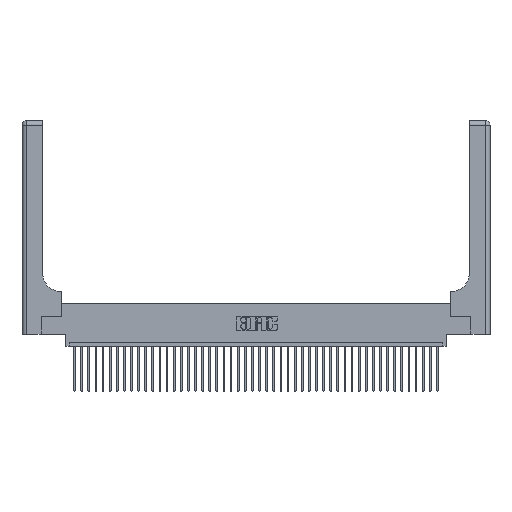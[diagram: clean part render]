
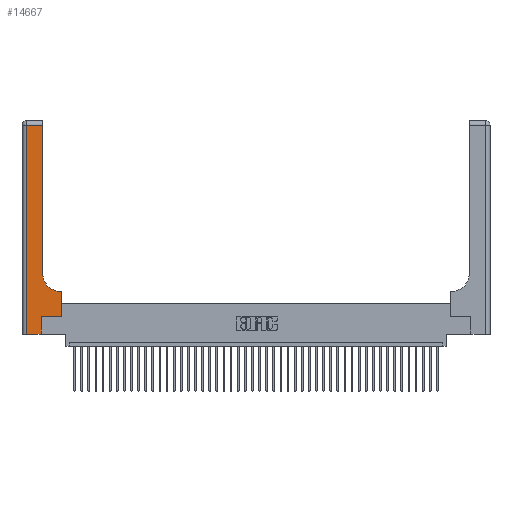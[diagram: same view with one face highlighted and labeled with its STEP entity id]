
A CAD part, top view. The second image highlights one B-rep face of the part: STEP entity #14667.
In plain terms, the highlighted planar face has unit normal (0, 0, 1).
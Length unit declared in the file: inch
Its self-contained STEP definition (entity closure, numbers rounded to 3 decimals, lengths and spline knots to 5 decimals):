
#72 = EDGE_CURVE ( 'NONE', #27932, #22813, #7140, .T. ) ;
#985 = CARTESIAN_POINT ( 'NONE',  ( 0.5585, 0.6, 0.37 ) ) ;
#1451 = VECTOR ( 'NONE', #40873, 39.37008 ) ;
#1504 = EDGE_CURVE ( 'NONE', #22813, #14280, #8619, .T. ) ;
#2608 = CARTESIAN_POINT ( 'NONE',  ( 0.5415, 0.6, 0.37 ) ) ;
#3847 = LINE ( 'NONE', #9476, #41307 ) ;
#5202 = EDGE_CURVE ( 'NONE', #39440, #27932, #33049, .T. ) ;
#6873 = CARTESIAN_POINT ( 'NONE',  ( 0.2915, 3., 0.37 ) ) ;
#7140 = CIRCLE ( 'NONE', #28200, 0.25 ) ;
#8091 = CARTESIAN_POINT ( 'NONE',  ( 0., 2.94, 0.37 ) ) ;
#8465 = DIRECTION ( 'NONE',  ( 1., 0., 0. ) ) ;
#8619 = LINE ( 'NONE', #6873, #30538 ) ;
#9246 = DIRECTION ( 'NONE',  ( 0., 1., 0. ) ) ;
#9343 = CARTESIAN_POINT ( 'NONE',  ( 0.5585, 0.25, 0.37 ) ) ;
#9476 = CARTESIAN_POINT ( 'NONE',  ( 0.5585, 0.25, 0.37 ) ) ;
#10538 = EDGE_LOOP ( 'NONE', ( #39473, #32038, #26495, #14213, #32783, #10696, #21372, #36555, #38969 ) ) ;
#10696 = ORIENTED_EDGE ( 'NONE', *, *, #23498, .T. ) ;
#11428 = CARTESIAN_POINT ( 'NONE',  ( 0.2915, 0.85, 0.37 ) ) ;
#12403 = AXIS2_PLACEMENT_3D ( 'NONE', #36168, #19683, #12734 ) ;
#12734 = DIRECTION ( 'NONE',  ( -1., 0., 0. ) ) ;
#14213 = ORIENTED_EDGE ( 'NONE', *, *, #15661, .T. ) ;
#14280 = VERTEX_POINT ( 'NONE', #30694 ) ;
#14667 = ADVANCED_FACE ( 'NONE', ( #39148 ), #19255, .F. ) ;
#14731 = CARTESIAN_POINT ( 'NONE',  ( 0.06, 3., 0.37 ) ) ;
#14767 = VERTEX_POINT ( 'NONE', #30352 ) ;
#15527 = CARTESIAN_POINT ( 'NONE',  ( 0.269, 0., 0.37 ) ) ;
#15661 = EDGE_CURVE ( 'NONE', #36026, #15746, #40003, .T. ) ;
#15672 = LINE ( 'NONE', #8091, #42216 ) ;
#15746 = VERTEX_POINT ( 'NONE', #15527 ) ;
#15942 = CARTESIAN_POINT ( 'NONE',  ( 0.269, 0., 0.37 ) ) ;
#16786 = CARTESIAN_POINT ( 'NONE',  ( 0.2915, 0.6, 0.37 ) ) ;
#17571 = CARTESIAN_POINT ( 'NONE',  ( 0., 0., 0.37 ) ) ;
#18194 = EDGE_CURVE ( 'NONE', #37340, #39440, #3847, .T. ) ;
#18347 = VERTEX_POINT ( 'NONE', #23715 ) ;
#18417 = VECTOR ( 'NONE', #25386, 39.37008 ) ;
#18901 = VECTOR ( 'NONE', #8465, 39.37008 ) ;
#19255 = PLANE ( 'NONE',  #12403 ) ;
#19683 = DIRECTION ( 'NONE',  ( 0., 0., -1. ) ) ;
#20445 = CARTESIAN_POINT ( 'NONE',  ( 0.5415, 0.85, 0.37 ) ) ;
#21258 = LINE ( 'NONE', #15942, #41061 ) ;
#21372 = ORIENTED_EDGE ( 'NONE', *, *, #18194, .T. ) ;
#21979 = CARTESIAN_POINT ( 'NONE',  ( 0.269, 0.25, 0.37 ) ) ;
#22813 = VERTEX_POINT ( 'NONE', #11428 ) ;
#23498 = EDGE_CURVE ( 'NONE', #18347, #37340, #24638, .T. ) ;
#23715 = CARTESIAN_POINT ( 'NONE',  ( 0.269, 0.25, 0.37 ) ) ;
#24638 = LINE ( 'NONE', #21979, #18901 ) ;
#24661 = EDGE_CURVE ( 'NONE', #14280, #14767, #15672, .T. ) ;
#25351 = DIRECTION ( 'NONE',  ( 0., 1., 0. ) ) ;
#25386 = DIRECTION ( 'NONE',  ( 0., -1., 0. ) ) ;
#26143 = EDGE_CURVE ( 'NONE', #15746, #18347, #21258, .T. ) ;
#26495 = ORIENTED_EDGE ( 'NONE', *, *, #38997, .T. ) ;
#26892 = CARTESIAN_POINT ( 'NONE',  ( 0.06, 0., 0.37 ) ) ;
#27932 = VERTEX_POINT ( 'NONE', #2608 ) ;
#28200 = AXIS2_PLACEMENT_3D ( 'NONE', #20445, #34443, #30607 ) ;
#30349 = DIRECTION ( 'NONE',  ( -1., 0., 0. ) ) ;
#30352 = CARTESIAN_POINT ( 'NONE',  ( 0.06, 2.94, 0.37 ) ) ;
#30538 = VECTOR ( 'NONE', #40196, 39.37008 ) ;
#30607 = DIRECTION ( 'NONE',  ( 1., 0., 0. ) ) ;
#30694 = CARTESIAN_POINT ( 'NONE',  ( 0.2915, 2.94, 0.37 ) ) ;
#32038 = ORIENTED_EDGE ( 'NONE', *, *, #24661, .T. ) ;
#32783 = ORIENTED_EDGE ( 'NONE', *, *, #26143, .T. ) ;
#33049 = LINE ( 'NONE', #16786, #38227 ) ;
#34443 = DIRECTION ( 'NONE',  ( 0., 0., -1. ) ) ;
#34741 = DIRECTION ( 'NONE',  ( -1., 0., 0. ) ) ;
#36026 = VERTEX_POINT ( 'NONE', #26892 ) ;
#36168 = CARTESIAN_POINT ( 'NONE',  ( 0., 3., 0.37 ) ) ;
#36555 = ORIENTED_EDGE ( 'NONE', *, *, #5202, .T. ) ;
#36645 = LINE ( 'NONE', #14731, #18417 ) ;
#37340 = VERTEX_POINT ( 'NONE', #9343 ) ;
#38227 = VECTOR ( 'NONE', #30349, 39.37008 ) ;
#38969 = ORIENTED_EDGE ( 'NONE', *, *, #72, .T. ) ;
#38997 = EDGE_CURVE ( 'NONE', #14767, #36026, #36645, .T. ) ;
#39148 = FACE_OUTER_BOUND ( 'NONE', #10538, .T. ) ;
#39440 = VERTEX_POINT ( 'NONE', #985 ) ;
#39473 = ORIENTED_EDGE ( 'NONE', *, *, #1504, .T. ) ;
#40003 = LINE ( 'NONE', #17571, #1451 ) ;
#40196 = DIRECTION ( 'NONE',  ( 0., 1., 0. ) ) ;
#40873 = DIRECTION ( 'NONE',  ( 1., 0., 0. ) ) ;
#41061 = VECTOR ( 'NONE', #9246, 39.37008 ) ;
#41307 = VECTOR ( 'NONE', #25351, 39.37008 ) ;
#42216 = VECTOR ( 'NONE', #34741, 39.37008 ) ;
